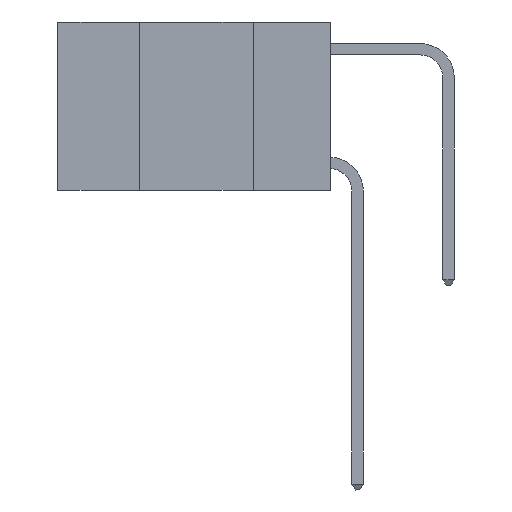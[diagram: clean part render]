
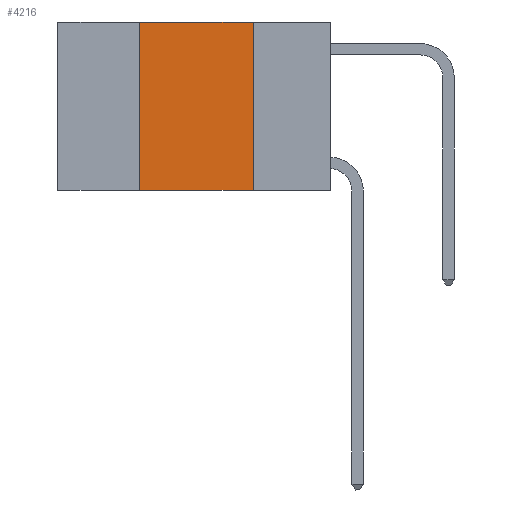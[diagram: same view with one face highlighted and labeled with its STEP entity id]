
A CAD part, left-side view. The second image highlights one B-rep face of the part: STEP entity #4216.
In plain terms, the highlighted planar face has unit normal (-1, 0, 0).
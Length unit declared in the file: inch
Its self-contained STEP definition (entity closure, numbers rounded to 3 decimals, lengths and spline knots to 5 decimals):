
#173 = VECTOR ( 'NONE', #8951, 39.37008 ) ;
#293 = PLANE ( 'NONE',  #10067 ) ;
#429 = ORIENTED_EDGE ( 'NONE', *, *, #4650, .T. ) ;
#698 = VERTEX_POINT ( 'NONE', #2896 ) ;
#738 = DIRECTION ( 'NONE',  ( 0., 0., 1. ) ) ;
#746 = VERTEX_POINT ( 'NONE', #7026 ) ;
#1645 = LINE ( 'NONE', #8304, #6047 ) ;
#1698 = CARTESIAN_POINT ( 'NONE',  ( 0., 0.42, 0. ) ) ;
#2024 = CARTESIAN_POINT ( 'NONE',  ( 0., 0.6, 0. ) ) ;
#2569 = EDGE_LOOP ( 'NONE', ( #4318, #2801, #6588, #429 ) ) ;
#2791 = FACE_OUTER_BOUND ( 'NONE', #2569, .T. ) ;
#2801 = ORIENTED_EDGE ( 'NONE', *, *, #6437, .F. ) ;
#2896 = CARTESIAN_POINT ( 'NONE',  ( 0., 0.17, -0.37 ) ) ;
#2966 = DIRECTION ( 'NONE',  ( 0., -1., 0. ) ) ;
#3059 = VECTOR ( 'NONE', #2966, 39.37008 ) ;
#3181 = LINE ( 'NONE', #9692, #173 ) ;
#3683 = CARTESIAN_POINT ( 'NONE',  ( 0., 0.17, 0. ) ) ;
#3767 = LINE ( 'NONE', #6975, #3059 ) ;
#4113 = EDGE_CURVE ( 'NONE', #6626, #746, #4928, .T. ) ;
#4132 = DIRECTION ( 'NONE',  ( 0., 0., -1. ) ) ;
#4216 = ADVANCED_FACE ( 'NONE', ( #2791 ), #293, .F. ) ;
#4318 = ORIENTED_EDGE ( 'NONE', *, *, #9628, .F. ) ;
#4650 = EDGE_CURVE ( 'NONE', #6626, #698, #3767, .T. ) ;
#4928 = LINE ( 'NONE', #1698, #5297 ) ;
#5297 = VECTOR ( 'NONE', #738, 39.37008 ) ;
#6047 = VECTOR ( 'NONE', #4132, 39.37008 ) ;
#6437 = EDGE_CURVE ( 'NONE', #746, #8965, #3181, .T. ) ;
#6588 = ORIENTED_EDGE ( 'NONE', *, *, #4113, .F. ) ;
#6626 = VERTEX_POINT ( 'NONE', #7068 ) ;
#6975 = CARTESIAN_POINT ( 'NONE',  ( 0., 0.6, -0.37 ) ) ;
#7026 = CARTESIAN_POINT ( 'NONE',  ( 0., 0.42, 0. ) ) ;
#7068 = CARTESIAN_POINT ( 'NONE',  ( 0., 0.42, -0.37 ) ) ;
#7771 = DIRECTION ( 'NONE',  ( 1., 0., 0. ) ) ;
#8304 = CARTESIAN_POINT ( 'NONE',  ( 0., 0.17, 0. ) ) ;
#8951 = DIRECTION ( 'NONE',  ( 0., -1., 0. ) ) ;
#8965 = VERTEX_POINT ( 'NONE', #3683 ) ;
#9295 = DIRECTION ( 'NONE',  ( 0., 0., -1. ) ) ;
#9628 = EDGE_CURVE ( 'NONE', #8965, #698, #1645, .T. ) ;
#9692 = CARTESIAN_POINT ( 'NONE',  ( 0., 0.6, 0. ) ) ;
#10067 = AXIS2_PLACEMENT_3D ( 'NONE', #2024, #7771, #9295 ) ;
